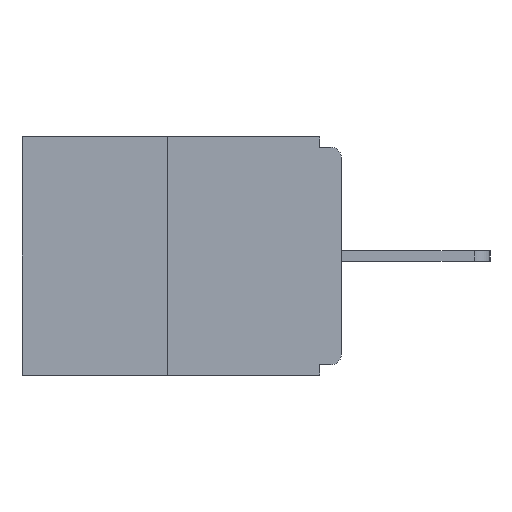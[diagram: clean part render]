
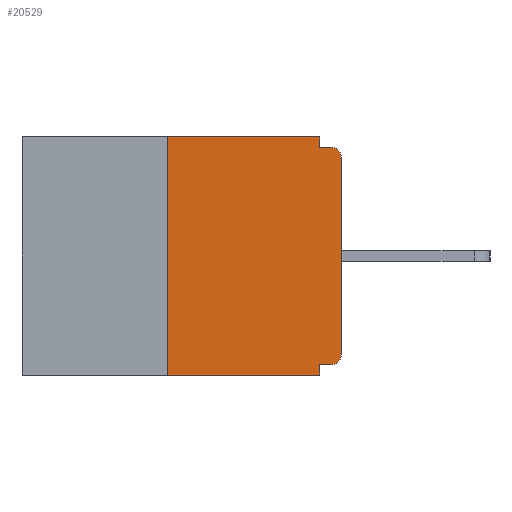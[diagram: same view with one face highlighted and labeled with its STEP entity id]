
A CAD part, left-side view. The second image highlights one B-rep face of the part: STEP entity #20529.
In plain terms, the highlighted planar face has unit normal (-1, 0, 0).
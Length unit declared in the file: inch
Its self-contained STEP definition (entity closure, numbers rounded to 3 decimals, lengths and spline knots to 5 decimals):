
#95 = LINE ( 'NONE', #10426, #4878 ) ;
#397 = CARTESIAN_POINT ( 'NONE',  ( 0., 0.031, -0.343 ) ) ;
#567 = DIRECTION ( 'NONE',  ( 0., 1., 0. ) ) ;
#680 = VERTEX_POINT ( 'NONE', #24702 ) ;
#1673 = DIRECTION ( 'NONE',  ( 0., -1., 0. ) ) ;
#1804 = DIRECTION ( 'NONE',  ( 0., 0., -1. ) ) ;
#1858 = CARTESIAN_POINT ( 'NONE',  ( 0., 0.46, 0. ) ) ;
#2017 = VERTEX_POINT ( 'NONE', #16130 ) ;
#2213 = VERTEX_POINT ( 'NONE', #3175 ) ;
#2230 = CARTESIAN_POINT ( 'NONE',  ( 0., 0.031, -0.343 ) ) ;
#2285 = EDGE_CURVE ( 'NONE', #14190, #9668, #12546, .T. ) ;
#2337 = CARTESIAN_POINT ( 'NONE',  ( 0., 0., -0.313 ) ) ;
#2904 = VECTOR ( 'NONE', #9292, 39.37008 ) ;
#2918 = VECTOR ( 'NONE', #21726, 39.37008 ) ;
#3175 = CARTESIAN_POINT ( 'NONE',  ( 0., 0.25, -0.343 ) ) ;
#3908 = DIRECTION ( 'NONE',  ( 0., 0., -1. ) ) ;
#4041 = VERTEX_POINT ( 'NONE', #22916 ) ;
#4205 = LINE ( 'NONE', #19887, #2918 ) ;
#4303 = EDGE_CURVE ( 'NONE', #2017, #680, #18513, .T. ) ;
#4736 = CARTESIAN_POINT ( 'NONE',  ( 0., 0.015, -0.313 ) ) ;
#4878 = VECTOR ( 'NONE', #567, 39.37008 ) ;
#5681 = EDGE_CURVE ( 'NONE', #12567, #22793, #13277, .T. ) ;
#5693 = DIRECTION ( 'NONE',  ( 0., 0., -1. ) ) ;
#5886 = PLANE ( 'NONE',  #17172 ) ;
#5983 = DIRECTION ( 'NONE',  ( -1., 0., 0. ) ) ;
#6891 = CIRCLE ( 'NONE', #15257, 0.015 ) ;
#7000 = EDGE_CURVE ( 'NONE', #2213, #22793, #18793, .T. ) ;
#7311 = DIRECTION ( 'NONE',  ( 0., -1., 0. ) ) ;
#7365 = DIRECTION ( 'NONE',  ( 0., -1., 0. ) ) ;
#7678 = EDGE_CURVE ( 'NONE', #680, #17177, #18463, .T. ) ;
#8806 = VERTEX_POINT ( 'NONE', #8957 ) ;
#8821 = FACE_OUTER_BOUND ( 'NONE', #9459, .T. ) ;
#8865 = CARTESIAN_POINT ( 'NONE',  ( 0., 0.031, 0. ) ) ;
#8957 = CARTESIAN_POINT ( 'NONE',  ( 0., 0.25, 0. ) ) ;
#9292 = DIRECTION ( 'NONE',  ( 0., 0., -1. ) ) ;
#9459 = EDGE_LOOP ( 'NONE', ( #20503, #20446, #20526, #16476, #19176, #19245, #13311, #13287, #15083, #14530 ) ) ;
#9483 = AXIS2_PLACEMENT_3D ( 'NONE', #4736, #5983, #5693 ) ;
#9517 = EDGE_CURVE ( 'NONE', #2213, #8806, #23003, .T. ) ;
#9668 = VERTEX_POINT ( 'NONE', #2337 ) ;
#10426 = CARTESIAN_POINT ( 'NONE',  ( 0., 0., -0.328 ) ) ;
#10593 = CARTESIAN_POINT ( 'NONE',  ( 0., 0.015, -0.328 ) ) ;
#11463 = DIRECTION ( 'NONE',  ( -1., 0., 0. ) ) ;
#12048 = VECTOR ( 'NONE', #1804, 39.37008 ) ;
#12546 = CIRCLE ( 'NONE', #9483, 0.015 ) ;
#12567 = VERTEX_POINT ( 'NONE', #16447 ) ;
#12686 = VECTOR ( 'NONE', #7365, 39.37008 ) ;
#12878 = VECTOR ( 'NONE', #17546, 39.37008 ) ;
#13277 = LINE ( 'NONE', #2230, #12048 ) ;
#13287 = ORIENTED_EDGE ( 'NONE', *, *, #23164, .T. ) ;
#13311 = ORIENTED_EDGE ( 'NONE', *, *, #20570, .T. ) ;
#13465 = CARTESIAN_POINT ( 'NONE',  ( 0., 0.46, 0. ) ) ;
#13857 = EDGE_CURVE ( 'NONE', #8806, #2017, #16193, .T. ) ;
#14120 = EDGE_CURVE ( 'NONE', #14190, #12567, #95, .T. ) ;
#14190 = VERTEX_POINT ( 'NONE', #10593 ) ;
#14530 = ORIENTED_EDGE ( 'NONE', *, *, #4303, .F. ) ;
#15083 = ORIENTED_EDGE ( 'NONE', *, *, #7678, .F. ) ;
#15257 = AXIS2_PLACEMENT_3D ( 'NONE', #22891, #11463, #24762 ) ;
#15615 = DIRECTION ( 'NONE',  ( 1., 0., 0. ) ) ;
#16130 = CARTESIAN_POINT ( 'NONE',  ( 0., 0.031, 0. ) ) ;
#16193 = LINE ( 'NONE', #13465, #21772 ) ;
#16447 = CARTESIAN_POINT ( 'NONE',  ( 0., 0.031, -0.328 ) ) ;
#16476 = ORIENTED_EDGE ( 'NONE', *, *, #5681, .F. ) ;
#17172 = AXIS2_PLACEMENT_3D ( 'NONE', #1858, #15615, #3908 ) ;
#17177 = VERTEX_POINT ( 'NONE', #17671 ) ;
#17546 = DIRECTION ( 'NONE',  ( 0., 0., 1. ) ) ;
#17671 = CARTESIAN_POINT ( 'NONE',  ( 0., 0.015, -0.015 ) ) ;
#18463 = LINE ( 'NONE', #20828, #12686 ) ;
#18513 = LINE ( 'NONE', #8865, #2904 ) ;
#18793 = LINE ( 'NONE', #18891, #23743 ) ;
#18891 = CARTESIAN_POINT ( 'NONE',  ( 0., 0.46, -0.343 ) ) ;
#19176 = ORIENTED_EDGE ( 'NONE', *, *, #14120, .F. ) ;
#19245 = ORIENTED_EDGE ( 'NONE', *, *, #2285, .T. ) ;
#19887 = CARTESIAN_POINT ( 'NONE',  ( 0., 0., 0. ) ) ;
#20446 = ORIENTED_EDGE ( 'NONE', *, *, #9517, .F. ) ;
#20503 = ORIENTED_EDGE ( 'NONE', *, *, #13857, .F. ) ;
#20526 = ORIENTED_EDGE ( 'NONE', *, *, #7000, .T. ) ;
#20529 = ADVANCED_FACE ( 'NONE', ( #8821 ), #5886, .F. ) ;
#20570 = EDGE_CURVE ( 'NONE', #9668, #4041, #4205, .T. ) ;
#20828 = CARTESIAN_POINT ( 'NONE',  ( 0., 0., -0.015 ) ) ;
#21726 = DIRECTION ( 'NONE',  ( 0., 0., 1. ) ) ;
#21772 = VECTOR ( 'NONE', #1673, 39.37008 ) ;
#22793 = VERTEX_POINT ( 'NONE', #397 ) ;
#22891 = CARTESIAN_POINT ( 'NONE',  ( 0., 0.015, -0.03 ) ) ;
#22916 = CARTESIAN_POINT ( 'NONE',  ( 0., 0., -0.03 ) ) ;
#23003 = LINE ( 'NONE', #23064, #12878 ) ;
#23064 = CARTESIAN_POINT ( 'NONE',  ( 0., 0.25, 0. ) ) ;
#23164 = EDGE_CURVE ( 'NONE', #4041, #17177, #6891, .T. ) ;
#23743 = VECTOR ( 'NONE', #7311, 39.37008 ) ;
#24702 = CARTESIAN_POINT ( 'NONE',  ( 0., 0.031, -0.015 ) ) ;
#24762 = DIRECTION ( 'NONE',  ( 0., 0., -1. ) ) ;
